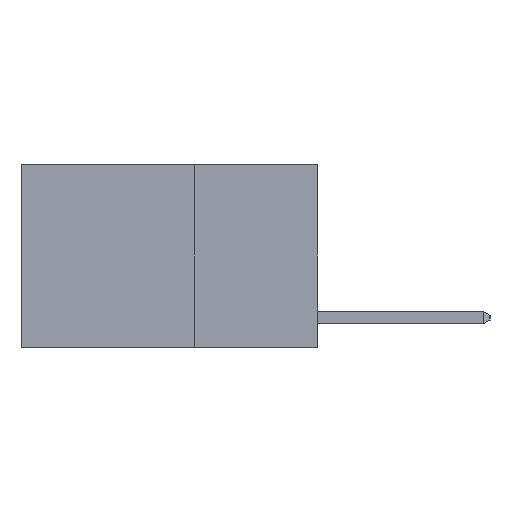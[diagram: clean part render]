
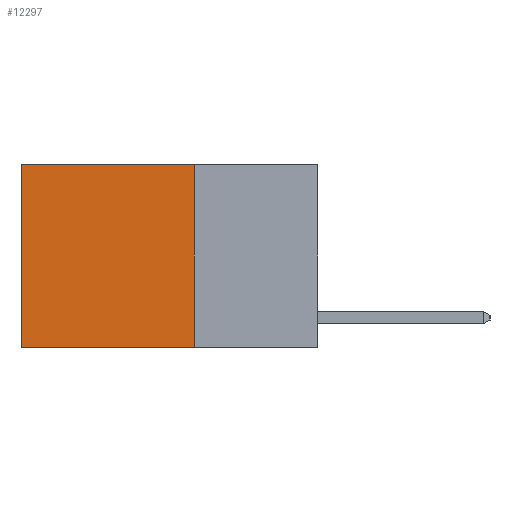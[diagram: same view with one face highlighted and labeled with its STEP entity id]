
A CAD part, left-side view. The second image highlights one B-rep face of the part: STEP entity #12297.
In plain terms, the highlighted planar face has unit normal (-1, 0, 0).
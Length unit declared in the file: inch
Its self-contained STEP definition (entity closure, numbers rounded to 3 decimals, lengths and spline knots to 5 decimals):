
#168 = CARTESIAN_POINT ( 'NONE',  ( 0.2625, 0.25, -0.37 ) ) ;
#407 = CARTESIAN_POINT ( 'NONE',  ( 0.2625, 0.6, 0. ) ) ;
#760 = EDGE_LOOP ( 'NONE', ( #2300, #3475, #1474, #7171 ) ) ;
#1060 = PLANE ( 'NONE',  #12765 ) ;
#1113 = DIRECTION ( 'NONE',  ( 1., 0., 0. ) ) ;
#1169 = VECTOR ( 'NONE', #10209, 39.37008 ) ;
#1474 = ORIENTED_EDGE ( 'NONE', *, *, #4266, .F. ) ;
#1625 = DIRECTION ( 'NONE',  ( 0., 0., -1. ) ) ;
#2300 = ORIENTED_EDGE ( 'NONE', *, *, #14415, .T. ) ;
#3013 = CARTESIAN_POINT ( 'NONE',  ( 0.2625, 0.25, 0. ) ) ;
#3475 = ORIENTED_EDGE ( 'NONE', *, *, #6157, .F. ) ;
#3616 = DIRECTION ( 'NONE',  ( 0., 1., 0. ) ) ;
#4266 = EDGE_CURVE ( 'NONE', #7479, #12206, #10087, .T. ) ;
#4812 = CARTESIAN_POINT ( 'NONE',  ( 0.2625, 0.6, -0.37 ) ) ;
#6157 = EDGE_CURVE ( 'NONE', #12206, #6563, #14702, .T. ) ;
#6338 = VERTEX_POINT ( 'NONE', #11485 ) ;
#6563 = VERTEX_POINT ( 'NONE', #4812 ) ;
#7171 = ORIENTED_EDGE ( 'NONE', *, *, #7262, .T. ) ;
#7216 = LINE ( 'NONE', #407, #9608 ) ;
#7262 = EDGE_CURVE ( 'NONE', #7479, #6338, #14155, .T. ) ;
#7479 = VERTEX_POINT ( 'NONE', #7589 ) ;
#7589 = CARTESIAN_POINT ( 'NONE',  ( 0.2625, 0.25, 0. ) ) ;
#7814 = VECTOR ( 'NONE', #9878, 39.37008 ) ;
#8408 = CARTESIAN_POINT ( 'NONE',  ( 0.2625, 0.25, 0. ) ) ;
#9605 = DIRECTION ( 'NONE',  ( 0., 0., -1. ) ) ;
#9608 = VECTOR ( 'NONE', #1625, 39.37008 ) ;
#9878 = DIRECTION ( 'NONE',  ( 0., 1., 0. ) ) ;
#10087 = LINE ( 'NONE', #3013, #1169 ) ;
#10209 = DIRECTION ( 'NONE',  ( 0., 0., -1. ) ) ;
#11104 = VECTOR ( 'NONE', #3616, 39.37008 ) ;
#11477 = CARTESIAN_POINT ( 'NONE',  ( 0.2625, 0.25, -0.37 ) ) ;
#11485 = CARTESIAN_POINT ( 'NONE',  ( 0.2625, 0.6, 0. ) ) ;
#11929 = FACE_OUTER_BOUND ( 'NONE', #760, .T. ) ;
#12206 = VERTEX_POINT ( 'NONE', #11477 ) ;
#12297 = ADVANCED_FACE ( 'NONE', ( #11929 ), #1060, .F. ) ;
#12765 = AXIS2_PLACEMENT_3D ( 'NONE', #13072, #1113, #9605 ) ;
#13072 = CARTESIAN_POINT ( 'NONE',  ( 0.2625, 0.25, 0. ) ) ;
#14155 = LINE ( 'NONE', #8408, #11104 ) ;
#14415 = EDGE_CURVE ( 'NONE', #6338, #6563, #7216, .T. ) ;
#14702 = LINE ( 'NONE', #168, #7814 ) ;
